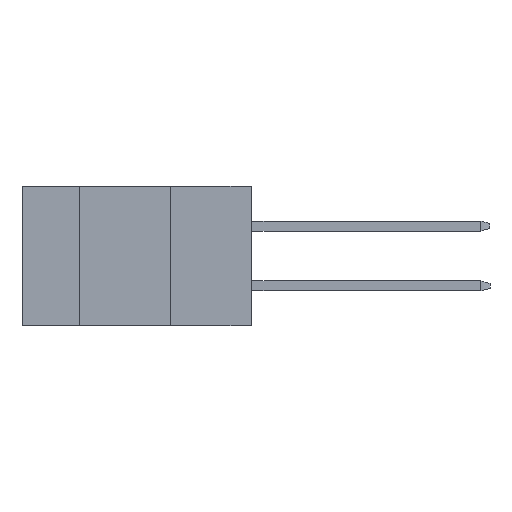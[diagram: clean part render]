
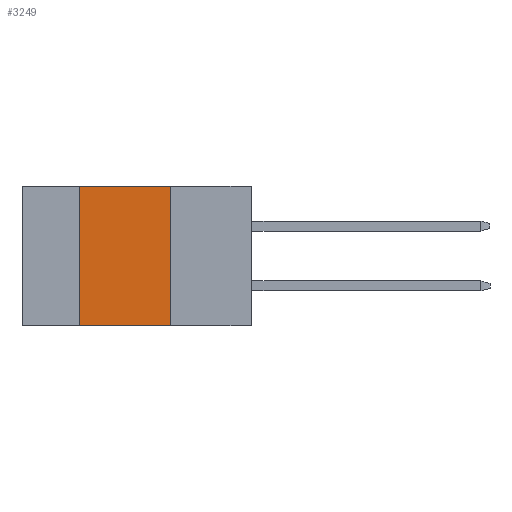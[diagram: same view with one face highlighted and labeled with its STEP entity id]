
A CAD part, left-side view. The second image highlights one B-rep face of the part: STEP entity #3249.
In plain terms, the highlighted planar face has unit normal (-1, 0, 0).
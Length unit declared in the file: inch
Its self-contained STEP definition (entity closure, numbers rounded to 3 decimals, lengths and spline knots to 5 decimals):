
#28 = CARTESIAN_POINT ( 'NONE',  ( 0., 0.72, 0. ) ) ;
#1650 = CARTESIAN_POINT ( 'NONE',  ( 0., 0.54, 0. ) ) ;
#2338 = VECTOR ( 'NONE', #2367, 39.37008 ) ;
#2367 = DIRECTION ( 'NONE',  ( 0., 0., 1. ) ) ;
#3249 = ADVANCED_FACE ( 'NONE', ( #5345 ), #10786, .F. ) ;
#3511 = CARTESIAN_POINT ( 'NONE',  ( 0., 0.54, -0.437 ) ) ;
#3542 = EDGE_LOOP ( 'NONE', ( #4455, #3784, #11283, #9708 ) ) ;
#3618 = DIRECTION ( 'NONE',  ( 0., 0., -1. ) ) ;
#3784 = ORIENTED_EDGE ( 'NONE', *, *, #5535, .F. ) ;
#4109 = LINE ( 'NONE', #28, #13873 ) ;
#4455 = ORIENTED_EDGE ( 'NONE', *, *, #16791, .F. ) ;
#4726 = DIRECTION ( 'NONE',  ( 0., 0., -1. ) ) ;
#4966 = CARTESIAN_POINT ( 'NONE',  ( 0., 0.254, -0.437 ) ) ;
#5345 = FACE_OUTER_BOUND ( 'NONE', #3542, .T. ) ;
#5535 = EDGE_CURVE ( 'NONE', #15344, #12814, #4109, .T. ) ;
#6315 = LINE ( 'NONE', #4966, #8265 ) ;
#6930 = VECTOR ( 'NONE', #16389, 39.37008 ) ;
#6979 = CARTESIAN_POINT ( 'NONE',  ( 0., 0.72, -0.437 ) ) ;
#8136 = CARTESIAN_POINT ( 'NONE',  ( 0., 0.72, 0. ) ) ;
#8223 = DIRECTION ( 'NONE',  ( 0., -1., 0. ) ) ;
#8265 = VECTOR ( 'NONE', #3618, 39.37008 ) ;
#9708 = ORIENTED_EDGE ( 'NONE', *, *, #12641, .T. ) ;
#9755 = VERTEX_POINT ( 'NONE', #11096 ) ;
#10494 = CARTESIAN_POINT ( 'NONE',  ( 0., 0.254, 0. ) ) ;
#10786 = PLANE ( 'NONE',  #15384 ) ;
#11059 = LINE ( 'NONE', #6979, #6930 ) ;
#11096 = CARTESIAN_POINT ( 'NONE',  ( 0., 0.54, -0.437 ) ) ;
#11116 = EDGE_CURVE ( 'NONE', #9755, #15344, #11528, .T. ) ;
#11283 = ORIENTED_EDGE ( 'NONE', *, *, #11116, .F. ) ;
#11528 = LINE ( 'NONE', #3511, #2338 ) ;
#12641 = EDGE_CURVE ( 'NONE', #9755, #15557, #11059, .T. ) ;
#12814 = VERTEX_POINT ( 'NONE', #10494 ) ;
#13536 = DIRECTION ( 'NONE',  ( 1., 0., 0. ) ) ;
#13873 = VECTOR ( 'NONE', #8223, 39.37008 ) ;
#15344 = VERTEX_POINT ( 'NONE', #1650 ) ;
#15384 = AXIS2_PLACEMENT_3D ( 'NONE', #8136, #13536, #4726 ) ;
#15557 = VERTEX_POINT ( 'NONE', #15957 ) ;
#15957 = CARTESIAN_POINT ( 'NONE',  ( 0., 0.254, -0.437 ) ) ;
#16389 = DIRECTION ( 'NONE',  ( 0., -1., 0. ) ) ;
#16791 = EDGE_CURVE ( 'NONE', #12814, #15557, #6315, .T. ) ;
